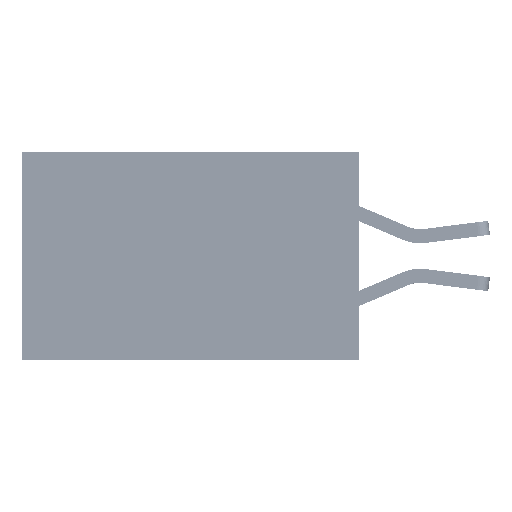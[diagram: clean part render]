
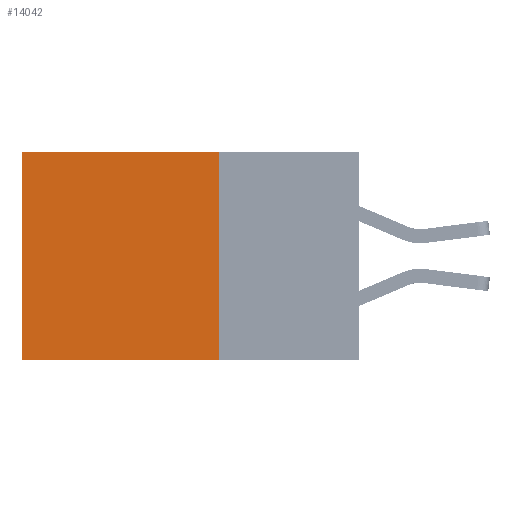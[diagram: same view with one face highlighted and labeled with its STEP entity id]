
A CAD part, left-side view. The second image highlights one B-rep face of the part: STEP entity #14042.
In plain terms, the highlighted planar face has unit normal (-1, 0, 0).
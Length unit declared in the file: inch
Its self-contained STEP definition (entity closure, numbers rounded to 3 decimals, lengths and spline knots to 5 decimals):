
#695 = LINE ( 'NONE', #34927, #5379 ) ;
#3675 = CARTESIAN_POINT ( 'NONE',  ( 0.2875, 0.25, 0. ) ) ;
#4953 = CARTESIAN_POINT ( 'NONE',  ( 0.2875, 0.25, -0.37 ) ) ;
#5203 = DIRECTION ( 'NONE',  ( 0., 0., -1. ) ) ;
#5379 = VECTOR ( 'NONE', #5203, 39.37008 ) ;
#5995 = LINE ( 'NONE', #29644, #9150 ) ;
#8032 = CARTESIAN_POINT ( 'NONE',  ( 0.2875, 0.25, 0. ) ) ;
#8118 = VERTEX_POINT ( 'NONE', #40128 ) ;
#8397 = VERTEX_POINT ( 'NONE', #15574 ) ;
#9150 = VECTOR ( 'NONE', #15975, 39.37008 ) ;
#10329 = VECTOR ( 'NONE', #37493, 39.37008 ) ;
#11075 = PLANE ( 'NONE',  #20610 ) ;
#11503 = DIRECTION ( 'NONE',  ( 0., 0., -1. ) ) ;
#11812 = CARTESIAN_POINT ( 'NONE',  ( 0.2875, 0.6, 0. ) ) ;
#11870 = VERTEX_POINT ( 'NONE', #11812 ) ;
#14042 = ADVANCED_FACE ( 'NONE', ( #34287 ), #11075, .F. ) ;
#14336 = EDGE_CURVE ( 'NONE', #15109, #11870, #16254, .T. ) ;
#15109 = VERTEX_POINT ( 'NONE', #41934 ) ;
#15574 = CARTESIAN_POINT ( 'NONE',  ( 0.2875, 0.6, -0.37 ) ) ;
#15975 = DIRECTION ( 'NONE',  ( 0., 0., -1. ) ) ;
#16254 = LINE ( 'NONE', #3675, #21220 ) ;
#16820 = EDGE_CURVE ( 'NONE', #11870, #8397, #695, .T. ) ;
#19777 = EDGE_CURVE ( 'NONE', #8118, #8397, #31001, .T. ) ;
#20610 = AXIS2_PLACEMENT_3D ( 'NONE', #8032, #40586, #11503 ) ;
#21220 = VECTOR ( 'NONE', #37445, 39.37008 ) ;
#25079 = ORIENTED_EDGE ( 'NONE', *, *, #19777, .F. ) ;
#28504 = ORIENTED_EDGE ( 'NONE', *, *, #41025, .F. ) ;
#29644 = CARTESIAN_POINT ( 'NONE',  ( 0.2875, 0.25, 0. ) ) ;
#31001 = LINE ( 'NONE', #4953, #10329 ) ;
#34287 = FACE_OUTER_BOUND ( 'NONE', #41687, .T. ) ;
#34927 = CARTESIAN_POINT ( 'NONE',  ( 0.2875, 0.6, 0. ) ) ;
#36364 = ORIENTED_EDGE ( 'NONE', *, *, #14336, .T. ) ;
#37410 = ORIENTED_EDGE ( 'NONE', *, *, #16820, .T. ) ;
#37445 = DIRECTION ( 'NONE',  ( 0., 1., 0. ) ) ;
#37493 = DIRECTION ( 'NONE',  ( 0., 1., 0. ) ) ;
#40128 = CARTESIAN_POINT ( 'NONE',  ( 0.2875, 0.25, -0.37 ) ) ;
#40586 = DIRECTION ( 'NONE',  ( 1., 0., 0. ) ) ;
#41025 = EDGE_CURVE ( 'NONE', #15109, #8118, #5995, .T. ) ;
#41687 = EDGE_LOOP ( 'NONE', ( #37410, #25079, #28504, #36364 ) ) ;
#41934 = CARTESIAN_POINT ( 'NONE',  ( 0.2875, 0.25, 0. ) ) ;
